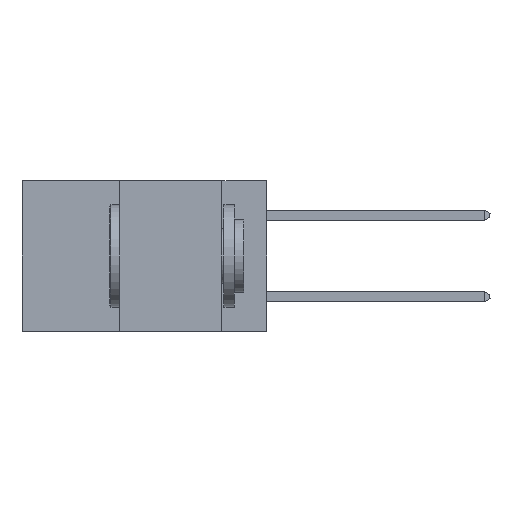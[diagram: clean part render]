
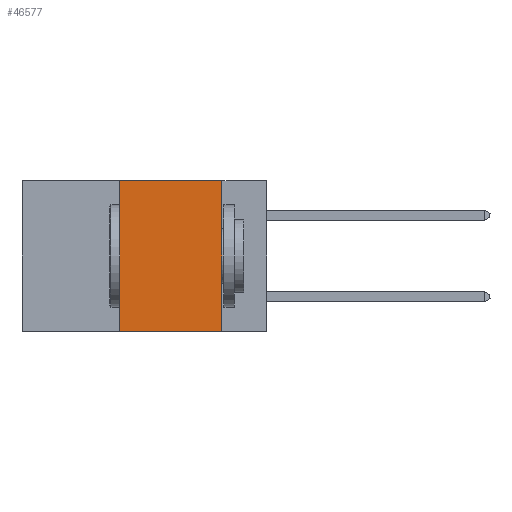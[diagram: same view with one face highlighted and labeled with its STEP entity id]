
A CAD part, left-side view. The second image highlights one B-rep face of the part: STEP entity #46577.
In plain terms, the highlighted planar face has unit normal (-1, 0, 0).
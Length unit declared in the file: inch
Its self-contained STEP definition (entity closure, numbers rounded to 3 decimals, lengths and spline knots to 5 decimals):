
#4975 = CARTESIAN_POINT ( 'NONE',  ( 0., 0.6, -0.37 ) ) ;
#5638 = DIRECTION ( 'NONE',  ( 0., -1., 0. ) ) ;
#6852 = CARTESIAN_POINT ( 'NONE',  ( 0., 0.11, 0. ) ) ;
#8687 = VECTOR ( 'NONE', #12868, 39.37008 ) ;
#9875 = DIRECTION ( 'NONE',  ( 1., 0., 0. ) ) ;
#11983 = LINE ( 'NONE', #50998, #47143 ) ;
#12489 = EDGE_CURVE ( 'NONE', #27412, #51791, #11983, .T. ) ;
#12868 = DIRECTION ( 'NONE',  ( 0., -1., 0. ) ) ;
#13307 = VECTOR ( 'NONE', #5638, 39.37008 ) ;
#13553 = DIRECTION ( 'NONE',  ( 0., 0., -1. ) ) ;
#14219 = ORIENTED_EDGE ( 'NONE', *, *, #39584, .T. ) ;
#15302 = ORIENTED_EDGE ( 'NONE', *, *, #47336, .F. ) ;
#17133 = FACE_OUTER_BOUND ( 'NONE', #45396, .T. ) ;
#19345 = LINE ( 'NONE', #4975, #8687 ) ;
#19613 = CARTESIAN_POINT ( 'NONE',  ( 0., 0.36, 0. ) ) ;
#20047 = CARTESIAN_POINT ( 'NONE',  ( 0., 0.36, -0.37 ) ) ;
#20421 = DIRECTION ( 'NONE',  ( 0., 0., -1. ) ) ;
#21875 = LINE ( 'NONE', #19613, #51456 ) ;
#25010 = VERTEX_POINT ( 'NONE', #32163 ) ;
#27412 = VERTEX_POINT ( 'NONE', #6852 ) ;
#27751 = LINE ( 'NONE', #29488, #13307 ) ;
#29488 = CARTESIAN_POINT ( 'NONE',  ( 0., 0.6, 0. ) ) ;
#32163 = CARTESIAN_POINT ( 'NONE',  ( 0., 0.36, 0. ) ) ;
#33420 = ORIENTED_EDGE ( 'NONE', *, *, #38856, .F. ) ;
#38336 = AXIS2_PLACEMENT_3D ( 'NONE', #46048, #9875, #13553 ) ;
#38856 = EDGE_CURVE ( 'NONE', #43643, #25010, #21875, .T. ) ;
#39584 = EDGE_CURVE ( 'NONE', #43643, #51791, #19345, .T. ) ;
#43643 = VERTEX_POINT ( 'NONE', #20047 ) ;
#45345 = PLANE ( 'NONE',  #38336 ) ;
#45396 = EDGE_LOOP ( 'NONE', ( #50922, #15302, #33420, #14219 ) ) ;
#46048 = CARTESIAN_POINT ( 'NONE',  ( 0., 0.6, 0. ) ) ;
#46577 = ADVANCED_FACE ( 'NONE', ( #17133 ), #45345, .F. ) ;
#47143 = VECTOR ( 'NONE', #20421, 39.37008 ) ;
#47336 = EDGE_CURVE ( 'NONE', #25010, #27412, #27751, .T. ) ;
#47711 = DIRECTION ( 'NONE',  ( 0., 0., 1. ) ) ;
#50012 = CARTESIAN_POINT ( 'NONE',  ( 0., 0.11, -0.37 ) ) ;
#50922 = ORIENTED_EDGE ( 'NONE', *, *, #12489, .F. ) ;
#50998 = CARTESIAN_POINT ( 'NONE',  ( 0., 0.11, 0. ) ) ;
#51456 = VECTOR ( 'NONE', #47711, 39.37008 ) ;
#51791 = VERTEX_POINT ( 'NONE', #50012 ) ;
